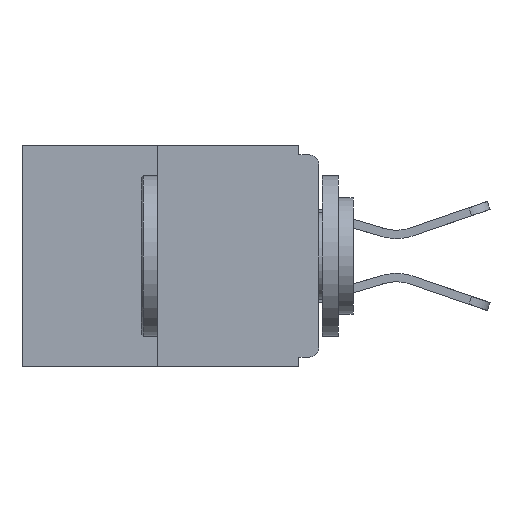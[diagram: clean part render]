
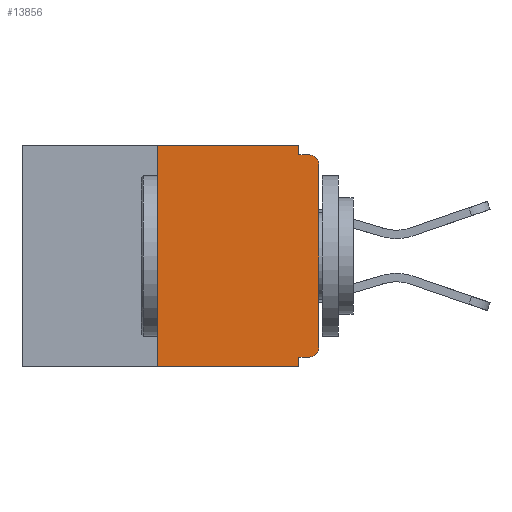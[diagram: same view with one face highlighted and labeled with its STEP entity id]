
A CAD part, left-side view. The second image highlights one B-rep face of the part: STEP entity #13856.
In plain terms, the highlighted planar face has unit normal (-1, 0, 0).
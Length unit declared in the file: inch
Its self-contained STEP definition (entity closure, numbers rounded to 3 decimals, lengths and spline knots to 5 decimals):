
#20 = DIRECTION ( 'NONE',  ( 0., 0., -1. ) ) ;
#135 = DIRECTION ( 'NONE',  ( -1., 0., 0. ) ) ;
#181 = ORIENTED_EDGE ( 'NONE', *, *, #8478, .T. ) ;
#293 = ORIENTED_EDGE ( 'NONE', *, *, #11812, .T. ) ;
#375 = LINE ( 'NONE', #8971, #4157 ) ;
#465 = VECTOR ( 'NONE', #9383, 39.37008 ) ;
#511 = CARTESIAN_POINT ( 'NONE',  ( 0., 0.031, 0. ) ) ;
#1059 = ORIENTED_EDGE ( 'NONE', *, *, #8597, .T. ) ;
#1114 = LINE ( 'NONE', #5374, #12405 ) ;
#1262 = EDGE_LOOP ( 'NONE', ( #14697, #16283, #293, #4885, #11376, #1059, #4690, #181, #10888, #1547 ) ) ;
#1493 = VERTEX_POINT ( 'NONE', #9565 ) ;
#1513 = EDGE_CURVE ( 'NONE', #7220, #13987, #7685, .T. ) ;
#1547 = ORIENTED_EDGE ( 'NONE', *, *, #6571, .F. ) ;
#1563 = CARTESIAN_POINT ( 'NONE',  ( 0., 0.031, -0.343 ) ) ;
#1865 = LINE ( 'NONE', #5612, #465 ) ;
#1880 = AXIS2_PLACEMENT_3D ( 'NONE', #16358, #11261, #20 ) ;
#2447 = CARTESIAN_POINT ( 'NONE',  ( 0., 0.25, 0. ) ) ;
#2542 = AXIS2_PLACEMENT_3D ( 'NONE', #6241, #135, #10193 ) ;
#2946 = VERTEX_POINT ( 'NONE', #14284 ) ;
#3062 = VERTEX_POINT ( 'NONE', #4328 ) ;
#3524 = DIRECTION ( 'NONE',  ( 0., 0., -1. ) ) ;
#4157 = VECTOR ( 'NONE', #15212, 39.37008 ) ;
#4328 = CARTESIAN_POINT ( 'NONE',  ( 0., 0.031, -0.343 ) ) ;
#4567 = DIRECTION ( 'NONE',  ( -1., 0., 0. ) ) ;
#4690 = ORIENTED_EDGE ( 'NONE', *, *, #1513, .T. ) ;
#4885 = ORIENTED_EDGE ( 'NONE', *, *, #13463, .F. ) ;
#4960 = VECTOR ( 'NONE', #8793, 39.37008 ) ;
#5230 = CARTESIAN_POINT ( 'NONE',  ( 0., 0., -0.03 ) ) ;
#5258 = CARTESIAN_POINT ( 'NONE',  ( 0., 0.015, -0.328 ) ) ;
#5374 = CARTESIAN_POINT ( 'NONE',  ( 0., 0.46, -0.343 ) ) ;
#5612 = CARTESIAN_POINT ( 'NONE',  ( 0., 0., -0.015 ) ) ;
#5712 = VECTOR ( 'NONE', #15934, 39.37008 ) ;
#6237 = VERTEX_POINT ( 'NONE', #7168 ) ;
#6241 = CARTESIAN_POINT ( 'NONE',  ( 0., 0.015, -0.313 ) ) ;
#6571 = EDGE_CURVE ( 'NONE', #1493, #12295, #11420, .T. ) ;
#6750 = DIRECTION ( 'NONE',  ( 0., -1., 0. ) ) ;
#6858 = CARTESIAN_POINT ( 'NONE',  ( 0., 0.46, 0. ) ) ;
#7141 = LINE ( 'NONE', #9864, #4960 ) ;
#7168 = CARTESIAN_POINT ( 'NONE',  ( 0., 0.25, -0.343 ) ) ;
#7220 = VERTEX_POINT ( 'NONE', #11078 ) ;
#7685 = LINE ( 'NONE', #15828, #5712 ) ;
#7755 = DIRECTION ( 'NONE',  ( 0., 0., -1. ) ) ;
#8478 = EDGE_CURVE ( 'NONE', #13987, #12403, #11551, .T. ) ;
#8597 = EDGE_CURVE ( 'NONE', #11781, #7220, #13721, .T. ) ;
#8793 = DIRECTION ( 'NONE',  ( 0., 0., 1. ) ) ;
#8971 = CARTESIAN_POINT ( 'NONE',  ( 0., 0., -0.328 ) ) ;
#9069 = VECTOR ( 'NONE', #9496, 39.37008 ) ;
#9383 = DIRECTION ( 'NONE',  ( 0., -1., 0. ) ) ;
#9496 = DIRECTION ( 'NONE',  ( 0., 0., -1. ) ) ;
#9565 = CARTESIAN_POINT ( 'NONE',  ( 0., 0.031, 0. ) ) ;
#9864 = CARTESIAN_POINT ( 'NONE',  ( 0., 0.25, 0. ) ) ;
#10193 = DIRECTION ( 'NONE',  ( 0., 0., -1. ) ) ;
#10272 = EDGE_CURVE ( 'NONE', #11781, #2946, #375, .T. ) ;
#10322 = DIRECTION ( 'NONE',  ( 0., -1., 0. ) ) ;
#10552 = VERTEX_POINT ( 'NONE', #2447 ) ;
#10888 = ORIENTED_EDGE ( 'NONE', *, *, #14134, .F. ) ;
#11078 = CARTESIAN_POINT ( 'NONE',  ( 0., 0., -0.313 ) ) ;
#11107 = AXIS2_PLACEMENT_3D ( 'NONE', #13308, #4567, #3524 ) ;
#11261 = DIRECTION ( 'NONE',  ( 1., 0., 0. ) ) ;
#11376 = ORIENTED_EDGE ( 'NONE', *, *, #10272, .F. ) ;
#11420 = LINE ( 'NONE', #511, #9069 ) ;
#11551 = CIRCLE ( 'NONE', #11107, 0.015 ) ;
#11769 = VECTOR ( 'NONE', #7755, 39.37008 ) ;
#11781 = VERTEX_POINT ( 'NONE', #5258 ) ;
#11812 = EDGE_CURVE ( 'NONE', #6237, #3062, #1114, .T. ) ;
#12163 = FACE_OUTER_BOUND ( 'NONE', #1262, .T. ) ;
#12295 = VERTEX_POINT ( 'NONE', #14669 ) ;
#12340 = LINE ( 'NONE', #1563, #11769 ) ;
#12403 = VERTEX_POINT ( 'NONE', #15162 ) ;
#12405 = VECTOR ( 'NONE', #10322, 39.37008 ) ;
#12449 = EDGE_CURVE ( 'NONE', #10552, #1493, #14367, .T. ) ;
#13308 = CARTESIAN_POINT ( 'NONE',  ( 0., 0.015, -0.03 ) ) ;
#13463 = EDGE_CURVE ( 'NONE', #2946, #3062, #12340, .T. ) ;
#13721 = CIRCLE ( 'NONE', #2542, 0.015 ) ;
#13810 = PLANE ( 'NONE',  #1880 ) ;
#13856 = ADVANCED_FACE ( 'NONE', ( #12163 ), #13810, .F. ) ;
#13967 = VECTOR ( 'NONE', #6750, 39.37008 ) ;
#13987 = VERTEX_POINT ( 'NONE', #5230 ) ;
#14134 = EDGE_CURVE ( 'NONE', #12295, #12403, #1865, .T. ) ;
#14284 = CARTESIAN_POINT ( 'NONE',  ( 0., 0.031, -0.328 ) ) ;
#14367 = LINE ( 'NONE', #6858, #13967 ) ;
#14669 = CARTESIAN_POINT ( 'NONE',  ( 0., 0.031, -0.015 ) ) ;
#14697 = ORIENTED_EDGE ( 'NONE', *, *, #12449, .F. ) ;
#15162 = CARTESIAN_POINT ( 'NONE',  ( 0., 0.015, -0.015 ) ) ;
#15212 = DIRECTION ( 'NONE',  ( 0., 1., 0. ) ) ;
#15736 = EDGE_CURVE ( 'NONE', #6237, #10552, #7141, .T. ) ;
#15828 = CARTESIAN_POINT ( 'NONE',  ( 0., 0., 0. ) ) ;
#15934 = DIRECTION ( 'NONE',  ( 0., 0., 1. ) ) ;
#16283 = ORIENTED_EDGE ( 'NONE', *, *, #15736, .F. ) ;
#16358 = CARTESIAN_POINT ( 'NONE',  ( 0., 0.46, 0. ) ) ;
